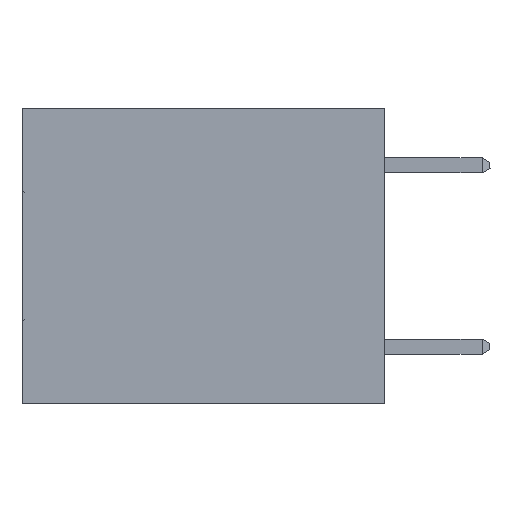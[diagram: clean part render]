
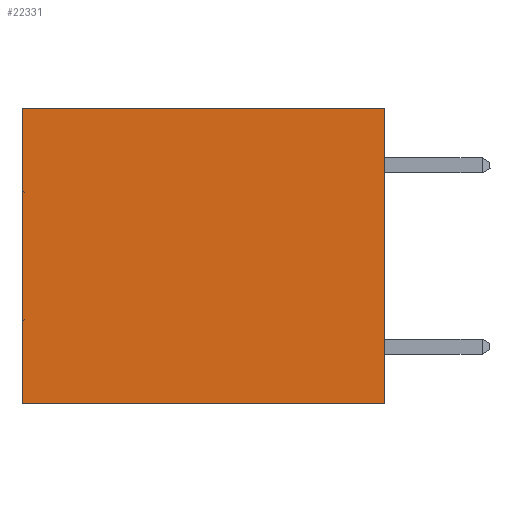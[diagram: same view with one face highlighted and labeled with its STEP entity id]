
A CAD part, left-side view. The second image highlights one B-rep face of the part: STEP entity #22331.
In plain terms, the highlighted planar face has unit normal (-1, 0, 0).
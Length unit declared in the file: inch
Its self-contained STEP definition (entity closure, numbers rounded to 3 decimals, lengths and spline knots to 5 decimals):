
#1831 = LINE ( 'NONE', #26464, #17907 ) ;
#5072 = CARTESIAN_POINT ( 'NONE',  ( 0.3165, 0., -0.49 ) ) ;
#5080 = VERTEX_POINT ( 'NONE', #25755 ) ;
#7433 = CARTESIAN_POINT ( 'NONE',  ( 0.3165, 0., -0.49 ) ) ;
#7503 = VERTEX_POINT ( 'NONE', #5072 ) ;
#7684 = DIRECTION ( 'NONE',  ( 0., 1., 0. ) ) ;
#8156 = CARTESIAN_POINT ( 'NONE',  ( 0.3165, 0.6, -0.49 ) ) ;
#8415 = ORIENTED_EDGE ( 'NONE', *, *, #28230, .T. ) ;
#9007 = LINE ( 'NONE', #7433, #13806 ) ;
#11091 = CARTESIAN_POINT ( 'NONE',  ( 0.3165, 0., -0.49 ) ) ;
#11095 = ORIENTED_EDGE ( 'NONE', *, *, #35997, .F. ) ;
#11867 = DIRECTION ( 'NONE',  ( 0., 0., -1. ) ) ;
#13806 = VECTOR ( 'NONE', #7684, 39.37008 ) ;
#13836 = VERTEX_POINT ( 'NONE', #8156 ) ;
#14636 = VECTOR ( 'NONE', #28565, 39.37008 ) ;
#15290 = EDGE_CURVE ( 'NONE', #5080, #25817, #1831, .T. ) ;
#15918 = LINE ( 'NONE', #11091, #14636 ) ;
#17907 = VECTOR ( 'NONE', #30136, 39.37008 ) ;
#18625 = CARTESIAN_POINT ( 'NONE',  ( 0.3165, 0.6, -0.49 ) ) ;
#20117 = DIRECTION ( 'NONE',  ( 1., 0., 0. ) ) ;
#20889 = EDGE_LOOP ( 'NONE', ( #8415, #27093, #11095, #23677 ) ) ;
#21283 = VECTOR ( 'NONE', #32892, 39.37008 ) ;
#22331 = ADVANCED_FACE ( 'NONE', ( #29114 ), #31677, .F. ) ;
#23677 = ORIENTED_EDGE ( 'NONE', *, *, #15290, .T. ) ;
#23771 = EDGE_CURVE ( 'NONE', #7503, #13836, #9007, .T. ) ;
#25755 = CARTESIAN_POINT ( 'NONE',  ( 0.3165, 0., 0. ) ) ;
#25817 = VERTEX_POINT ( 'NONE', #32758 ) ;
#26464 = CARTESIAN_POINT ( 'NONE',  ( 0.3165, 0., 0. ) ) ;
#27093 = ORIENTED_EDGE ( 'NONE', *, *, #23771, .F. ) ;
#28230 = EDGE_CURVE ( 'NONE', #25817, #13836, #29953, .T. ) ;
#28565 = DIRECTION ( 'NONE',  ( 0., 0., -1. ) ) ;
#29114 = FACE_OUTER_BOUND ( 'NONE', #20889, .T. ) ;
#29953 = LINE ( 'NONE', #18625, #21283 ) ;
#30136 = DIRECTION ( 'NONE',  ( 0., 1., 0. ) ) ;
#31677 = PLANE ( 'NONE',  #33264 ) ;
#32758 = CARTESIAN_POINT ( 'NONE',  ( 0.3165, 0.6, 0. ) ) ;
#32892 = DIRECTION ( 'NONE',  ( 0., 0., -1. ) ) ;
#33264 = AXIS2_PLACEMENT_3D ( 'NONE', #34613, #20117, #11867 ) ;
#34613 = CARTESIAN_POINT ( 'NONE',  ( 0.3165, 0., -0.49 ) ) ;
#35997 = EDGE_CURVE ( 'NONE', #5080, #7503, #15918, .T. ) ;
